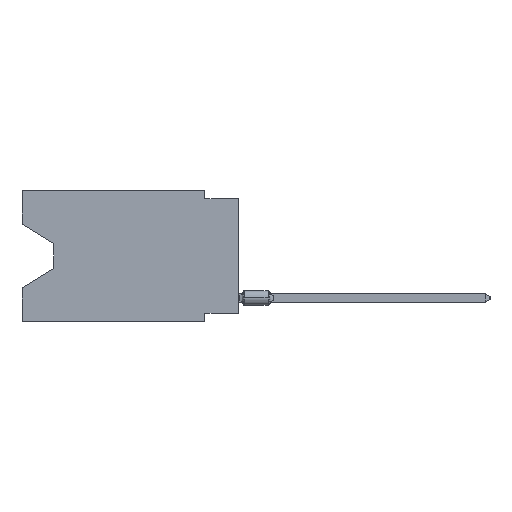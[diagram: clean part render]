
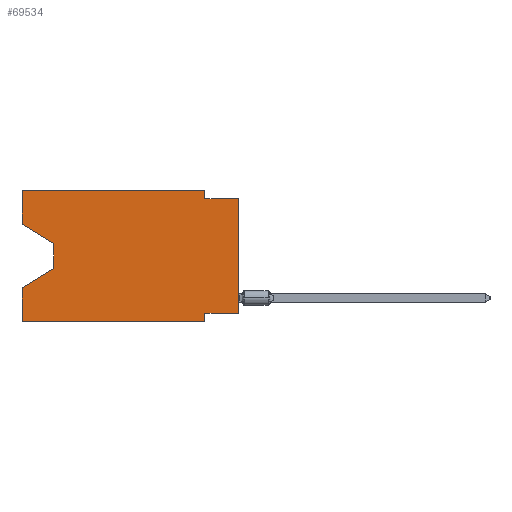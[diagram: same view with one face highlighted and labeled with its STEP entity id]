
A CAD part, left-side view. The second image highlights one B-rep face of the part: STEP entity #69534.
In plain terms, the highlighted planar face has unit normal (-1, 0, 0).
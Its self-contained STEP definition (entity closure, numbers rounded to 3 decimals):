
#588 = VECTOR ( 'NONE', #23381, 1000. ) ;
#1042 = VERTEX_POINT ( 'NONE', #43031 ) ;
#1095 = ORIENTED_EDGE ( 'NONE', *, *, #41800, .T. ) ;
#1326 = DIRECTION ( 'NONE',  ( 0., 0., -1. ) ) ;
#1729 = CARTESIAN_POINT ( 'NONE',  ( 0., 2.54, 0. ) ) ;
#2522 = CARTESIAN_POINT ( 'NONE',  ( 0., 13.97, -4.013 ) ) ;
#2724 = CARTESIAN_POINT ( 'NONE',  ( 0., 0., -9.271 ) ) ;
#2938 = CARTESIAN_POINT ( 'NONE',  ( 0., 16.383, 0. ) ) ;
#3443 = ORIENTED_EDGE ( 'NONE', *, *, #15845, .F. ) ;
#3596 = VECTOR ( 'NONE', #44070, 1000. ) ;
#5118 = VERTEX_POINT ( 'NONE', #61695 ) ;
#5245 = VECTOR ( 'NONE', #49954, 1000. ) ;
#5632 = CARTESIAN_POINT ( 'NONE',  ( 0., 2.54, -9.906 ) ) ;
#6669 = VECTOR ( 'NONE', #81523, 1000. ) ;
#6808 = DIRECTION ( 'NONE',  ( 0., 0., 1. ) ) ;
#6952 = ORIENTED_EDGE ( 'NONE', *, *, #28283, .T. ) ;
#7090 = VECTOR ( 'NONE', #61313, 1000. ) ;
#7994 = LINE ( 'NONE', #1729, #66975 ) ;
#8014 = CARTESIAN_POINT ( 'NONE',  ( 0., 16.383, -2.546 ) ) ;
#8675 = CARTESIAN_POINT ( 'NONE',  ( 0., 13.97, -5.893 ) ) ;
#8779 = FACE_OUTER_BOUND ( 'NONE', #79940, .T. ) ;
#10997 = ORIENTED_EDGE ( 'NONE', *, *, #72696, .F. ) ;
#12240 = CARTESIAN_POINT ( 'NONE',  ( 0., 2.54, -9.906 ) ) ;
#13217 = CARTESIAN_POINT ( 'NONE',  ( 0., 2.54, -9.271 ) ) ;
#15845 = EDGE_CURVE ( 'NONE', #5118, #1042, #51152, .T. ) ;
#17245 = EDGE_CURVE ( 'NONE', #79033, #41747, #65612, .T. ) ;
#17474 = LINE ( 'NONE', #42154, #56740 ) ;
#18025 = VECTOR ( 'NONE', #38166, 1000. ) ;
#23381 = DIRECTION ( 'NONE',  ( 0., 0., -1. ) ) ;
#23887 = DIRECTION ( 'NONE',  ( 0., 1., 0. ) ) ;
#24317 = ORIENTED_EDGE ( 'NONE', *, *, #32686, .F. ) ;
#25108 = VERTEX_POINT ( 'NONE', #5632 ) ;
#26275 = ORIENTED_EDGE ( 'NONE', *, *, #55737, .F. ) ;
#28046 = VERTEX_POINT ( 'NONE', #57481 ) ;
#28283 = EDGE_CURVE ( 'NONE', #44634, #43200, #57055, .T. ) ;
#28436 = DIRECTION ( 'NONE',  ( 0., 0., -1. ) ) ;
#28568 = EDGE_CURVE ( 'NONE', #28046, #41747, #69391, .T. ) ;
#30991 = LINE ( 'NONE', #64268, #38248 ) ;
#32686 = EDGE_CURVE ( 'NONE', #1042, #28046, #7994, .T. ) ;
#34423 = VERTEX_POINT ( 'NONE', #54169 ) ;
#34723 = PLANE ( 'NONE',  #74364 ) ;
#35122 = DIRECTION ( 'NONE',  ( 1., 0., 0. ) ) ;
#35124 = EDGE_CURVE ( 'NONE', #80063, #25108, #76182, .T. ) ;
#36003 = CARTESIAN_POINT ( 'NONE',  ( 0., 0., -0.635 ) ) ;
#38166 = DIRECTION ( 'NONE',  ( 0., 0., -1. ) ) ;
#38248 = VECTOR ( 'NONE', #23887, 1000. ) ;
#38723 = EDGE_CURVE ( 'NONE', #44634, #5118, #63893, .T. ) ;
#39253 = CARTESIAN_POINT ( 'NONE',  ( 0., 16.383, 0. ) ) ;
#39322 = CARTESIAN_POINT ( 'NONE',  ( 0., 0., 0. ) ) ;
#39886 = ORIENTED_EDGE ( 'NONE', *, *, #77806, .T. ) ;
#41747 = VERTEX_POINT ( 'NONE', #55933 ) ;
#41800 = EDGE_CURVE ( 'NONE', #34423, #25108, #17474, .T. ) ;
#42154 = CARTESIAN_POINT ( 'NONE',  ( 0., 16.383, -9.906 ) ) ;
#43031 = CARTESIAN_POINT ( 'NONE',  ( 0., 2.54, 0. ) ) ;
#43200 = VERTEX_POINT ( 'NONE', #73794 ) ;
#44070 = DIRECTION ( 'NONE',  ( 0., -1., 0. ) ) ;
#44634 = VERTEX_POINT ( 'NONE', #59128 ) ;
#45186 = CARTESIAN_POINT ( 'NONE',  ( 0., 13.97, -5.893 ) ) ;
#45194 = DIRECTION ( 'NONE',  ( 0., 0., 1. ) ) ;
#45235 = VECTOR ( 'NONE', #6808, 1000. ) ;
#46222 = ORIENTED_EDGE ( 'NONE', *, *, #38723, .F. ) ;
#48213 = VERTEX_POINT ( 'NONE', #69249 ) ;
#48474 = LINE ( 'NONE', #2522, #588 ) ;
#48596 = ORIENTED_EDGE ( 'NONE', *, *, #17245, .T. ) ;
#49954 = DIRECTION ( 'NONE',  ( 0., -0.855, -0.519 ) ) ;
#50729 = LINE ( 'NONE', #57399, #45235 ) ;
#51152 = LINE ( 'NONE', #69125, #3596 ) ;
#52528 = ORIENTED_EDGE ( 'NONE', *, *, #28568, .F. ) ;
#54169 = CARTESIAN_POINT ( 'NONE',  ( 0., 16.383, -9.906 ) ) ;
#55737 = EDGE_CURVE ( 'NONE', #79033, #80063, #30991, .T. ) ;
#55933 = CARTESIAN_POINT ( 'NONE',  ( 0., 0., -0.635 ) ) ;
#56740 = VECTOR ( 'NONE', #61764, 1000. ) ;
#56999 = VECTOR ( 'NONE', #45194, 1000. ) ;
#57055 = LINE ( 'NONE', #8014, #5245 ) ;
#57399 = CARTESIAN_POINT ( 'NONE',  ( 0., 16.383, 0. ) ) ;
#57481 = CARTESIAN_POINT ( 'NONE',  ( 0., 2.54, -0.635 ) ) ;
#59128 = CARTESIAN_POINT ( 'NONE',  ( 0., 16.383, -2.546 ) ) ;
#61313 = DIRECTION ( 'NONE',  ( 0., 0.855, -0.519 ) ) ;
#61695 = CARTESIAN_POINT ( 'NONE',  ( 0., 16.383, 0. ) ) ;
#61764 = DIRECTION ( 'NONE',  ( 0., -1., 0. ) ) ;
#63473 = DIRECTION ( 'NONE',  ( 0., 0., 1. ) ) ;
#63893 = LINE ( 'NONE', #39253, #74248 ) ;
#64268 = CARTESIAN_POINT ( 'NONE',  ( 0., 0., -9.271 ) ) ;
#65612 = LINE ( 'NONE', #39322, #56999 ) ;
#66760 = LINE ( 'NONE', #8675, #7090 ) ;
#66975 = VECTOR ( 'NONE', #1326, 1000. ) ;
#69125 = CARTESIAN_POINT ( 'NONE',  ( 0., 16.383, 0. ) ) ;
#69249 = CARTESIAN_POINT ( 'NONE',  ( 0., 16.383, -7.36 ) ) ;
#69391 = LINE ( 'NONE', #36003, #6669 ) ;
#69534 = ADVANCED_FACE ( 'NONE', ( #8779 ), #34723, .F. ) ;
#71016 = ORIENTED_EDGE ( 'NONE', *, *, #35124, .F. ) ;
#71489 = VERTEX_POINT ( 'NONE', #45186 ) ;
#72696 = EDGE_CURVE ( 'NONE', #34423, #48213, #50729, .T. ) ;
#73794 = CARTESIAN_POINT ( 'NONE',  ( 0., 13.97, -4.013 ) ) ;
#74248 = VECTOR ( 'NONE', #63473, 1000. ) ;
#74364 = AXIS2_PLACEMENT_3D ( 'NONE', #2938, #35122, #28436 ) ;
#74956 = ORIENTED_EDGE ( 'NONE', *, *, #78099, .T. ) ;
#76182 = LINE ( 'NONE', #12240, #18025 ) ;
#77806 = EDGE_CURVE ( 'NONE', #43200, #71489, #48474, .T. ) ;
#78099 = EDGE_CURVE ( 'NONE', #71489, #48213, #66760, .T. ) ;
#79033 = VERTEX_POINT ( 'NONE', #2724 ) ;
#79940 = EDGE_LOOP ( 'NONE', ( #6952, #39886, #74956, #10997, #1095, #71016, #26275, #48596, #52528, #24317, #3443, #46222 ) ) ;
#80063 = VERTEX_POINT ( 'NONE', #13217 ) ;
#81523 = DIRECTION ( 'NONE',  ( 0., -1., 0. ) ) ;
